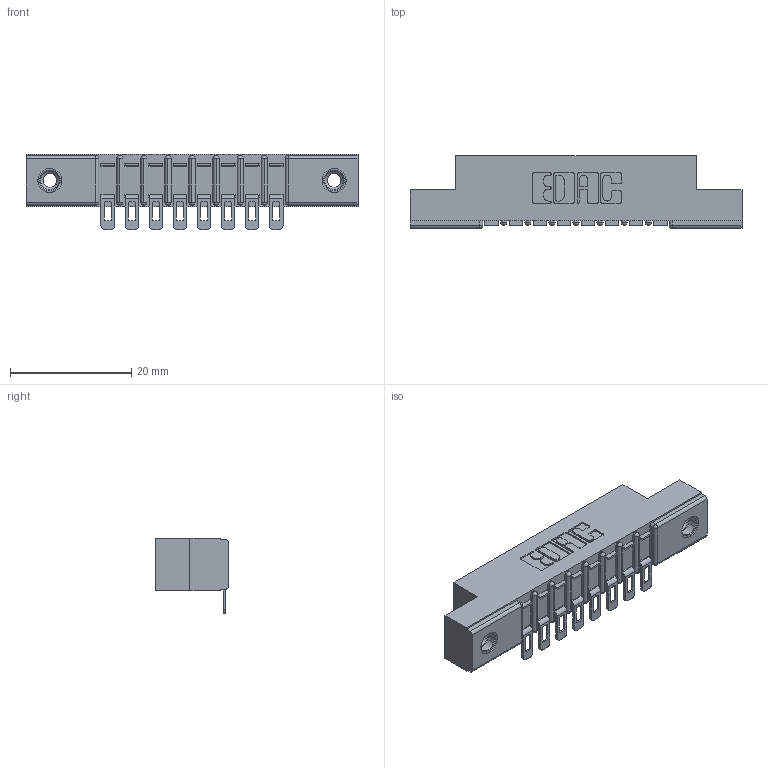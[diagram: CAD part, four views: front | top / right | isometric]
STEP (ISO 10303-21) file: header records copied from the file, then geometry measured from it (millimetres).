
FILE_DESCRIPTION (( 'STEP AP203' ), '1' );
FILE_NAME ('307-008-554-108.STEP', '2019-09-04T18:35:39', ( '' ), ( '' ), 'SwSTEP 2.0', 'SolidWorks 2016', '' );
FILE_SCHEMA (( 'CONFIG_CONTROL_DESIGN' ));
Length unit declared in the file: inch
Products named in the file (4): 345-250-001_345-250-003-102; 307-008-554-108; 307-290-002_554; 307 Part_.156 Dia Mounting Holes
Assembly tree (11 placements, depth 2):
  307-008-554-108
    307 Part_.156 Dia Mounting Holes
    307-290-002_554  x8
    345-250-001_345-250-003-102  x2
Bounding box: 54.71 x 12.01 x 12.52 mm (x, y, z)
Volume: 3601 mm3; surface area: 5822.8 mm2
Topology: 11 solids, 11 shells, 835 faces, 2483 edges, 1622 vertices
Faces by surface type: plane 470, cylinder 331, sphere 18, cone 12, torus 4
Entity records: 13200 total; most frequent: CARTESIAN_POINT 2201, ORIENTED_EDGE 2184, DIRECTION 2170, EDGE_CURVE 1092, VECTOR 812, LINE 812, VERTEX_POINT 710, AXIS2_PLACEMENT_3D 679
